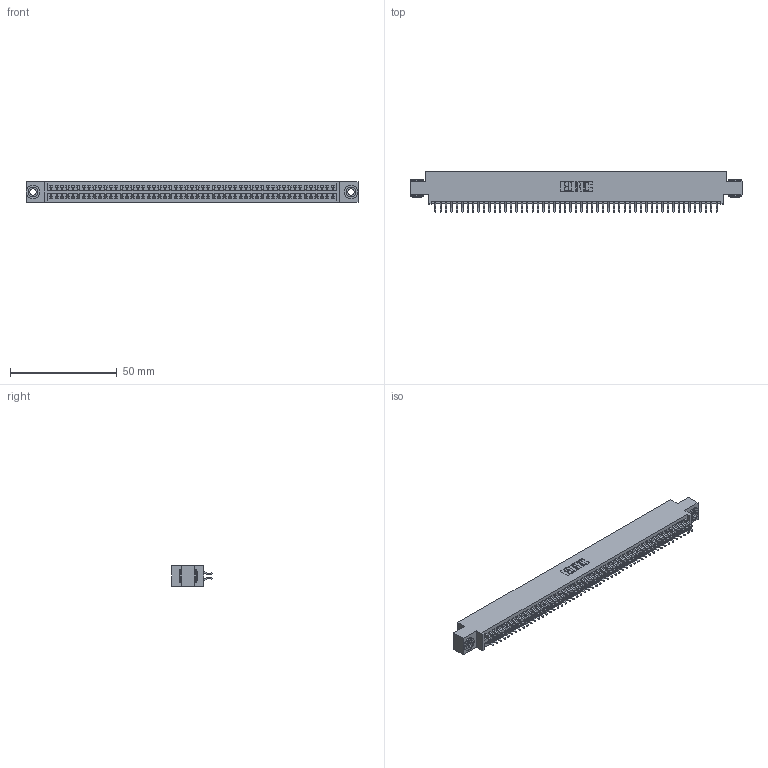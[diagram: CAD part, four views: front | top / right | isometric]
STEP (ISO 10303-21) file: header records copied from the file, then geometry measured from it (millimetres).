
FILE_DESCRIPTION (( 'STEP AP203' ), '1' );
FILE_NAME ('395-106-556-803.STEP', '2019-10-27T06:08:14', ( '' ), ( '' ), 'SwSTEP 2.0', 'SolidWorks 2016', '' );
FILE_SCHEMA (( 'CONFIG_CONTROL_DESIGN' ));
Length unit declared in the file: inch
Products named in the file (4): 395-106-556-803; 345 Part_0.170 Offset - 0.156 Dia-TH; 345-292-001_556 Tail; 345-250-002_345-250-002-102
Assembly tree (109 placements, depth 2):
  395-106-556-803
    345 Part_0.170 Offset - 0.156 Dia-TH
    345-292-001_556 Tail  x106
    345-250-002_345-250-002-102  x2
Bounding box: 155.83 x 19.24 x 9.4 mm (x, y, z)
Volume: 15141.3 mm3; surface area: 22850 mm2
Topology: 109 solids, 109 shells, 6104 faces, 18131 edges, 11942 vertices
Faces by surface type: plane 4016, cylinder 2080, cone 8
Entity records: 41106 total; most frequent: CARTESIAN_POINT 6871, ORIENTED_EDGE 6786, DIRECTION 6063, EDGE_CURVE 3393, LINE 3017, VECTOR 3017, VERTEX_POINT 2258, AXIS2_PLACEMENT_3D 1523
